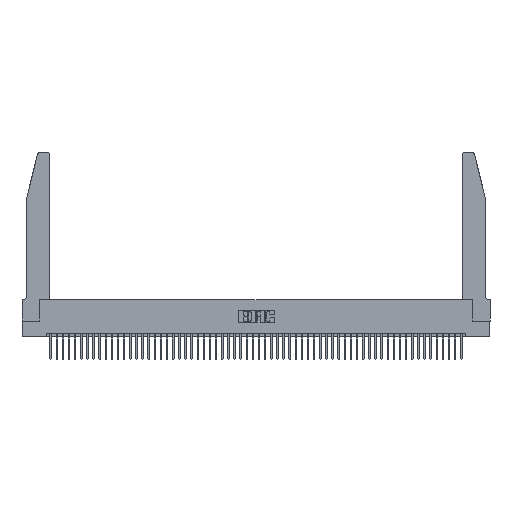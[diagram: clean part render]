
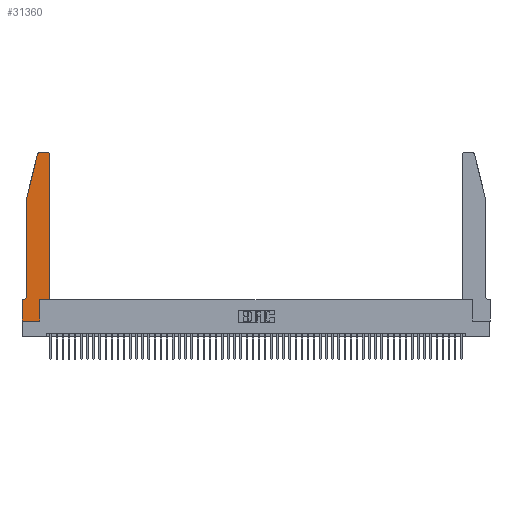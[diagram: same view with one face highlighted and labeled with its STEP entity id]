
A CAD part, top view. The second image highlights one B-rep face of the part: STEP entity #31360.
In plain terms, the highlighted planar face has unit normal (0, 0, 1).
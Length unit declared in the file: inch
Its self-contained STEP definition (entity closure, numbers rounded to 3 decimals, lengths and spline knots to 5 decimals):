
#433 = VERTEX_POINT ( 'NONE', #43734 ) ;
#1909 = ORIENTED_EDGE ( 'NONE', *, *, #45618, .T. ) ;
#3272 = FACE_OUTER_BOUND ( 'NONE', #50209, .T. ) ;
#3766 = CARTESIAN_POINT ( 'NONE',  ( 0., 0., 0.37 ) ) ;
#4046 = DIRECTION ( 'NONE',  ( 0., 0., -1. ) ) ;
#4512 = LINE ( 'NONE', #30137, #24346 ) ;
#6348 = CARTESIAN_POINT ( 'NONE',  ( 0.0755, 2., 0.37 ) ) ;
#7104 = ORIENTED_EDGE ( 'NONE', *, *, #36460, .T. ) ;
#7847 = ORIENTED_EDGE ( 'NONE', *, *, #46604, .T. ) ;
#8444 = VERTEX_POINT ( 'NONE', #13459 ) ;
#9307 = VERTEX_POINT ( 'NONE', #34593 ) ;
#9309 = VERTEX_POINT ( 'NONE', #9315 ) ;
#9315 = CARTESIAN_POINT ( 'NONE',  ( 0.4505, 2.72, 0.37 ) ) ;
#11654 = VECTOR ( 'NONE', #35386, 39.37008 ) ;
#12105 = CARTESIAN_POINT ( 'NONE',  ( 0.284, 2.72, 0.37 ) ) ;
#12354 = LINE ( 'NONE', #37042, #32099 ) ;
#13044 = CIRCLE ( 'NONE', #27682, 0.07 ) ;
#13131 = CARTESIAN_POINT ( 'NONE',  ( 0.0755, 0.42, 0.37 ) ) ;
#13279 = ORIENTED_EDGE ( 'NONE', *, *, #46031, .T. ) ;
#13411 = CARTESIAN_POINT ( 'NONE',  ( 0., 0.35, 0.37 ) ) ;
#13459 = CARTESIAN_POINT ( 'NONE',  ( 0.0055, 0.35, 0.37 ) ) ;
#13509 = VERTEX_POINT ( 'NONE', #30182 ) ;
#14500 = CARTESIAN_POINT ( 'NONE',  ( 0.0755, 2., 0.37 ) ) ;
#14809 = CARTESIAN_POINT ( 'NONE',  ( 0., 0.35, 0.37 ) ) ;
#15354 = CIRCLE ( 'NONE', #24052, 0.03 ) ;
#15947 = LINE ( 'NONE', #53700, #48142 ) ;
#16117 = VERTEX_POINT ( 'NONE', #13131 ) ;
#16398 = DIRECTION ( 'NONE',  ( 1., 0., 0. ) ) ;
#17686 = DIRECTION ( 'NONE',  ( 1., 0., 0. ) ) ;
#17772 = ORIENTED_EDGE ( 'NONE', *, *, #32910, .T. ) ;
#17981 = ORIENTED_EDGE ( 'NONE', *, *, #23582, .T. ) ;
#18593 = DIRECTION ( 'NONE',  ( 0., -1., 0. ) ) ;
#20157 = VERTEX_POINT ( 'NONE', #3766 ) ;
#20352 = LINE ( 'NONE', #6348, #41393 ) ;
#20749 = EDGE_CURVE ( 'NONE', #8444, #48089, #12354, .T. ) ;
#20758 = DIRECTION ( 'NONE',  ( 0., 1., 0. ) ) ;
#21762 = VERTEX_POINT ( 'NONE', #31262 ) ;
#21890 = CARTESIAN_POINT ( 'NONE',  ( 0.4205, 2.72, 0.37 ) ) ;
#22888 = LINE ( 'NONE', #31159, #11654 ) ;
#23380 = DIRECTION ( 'NONE',  ( -0.239, -0.971, 0. ) ) ;
#23582 = EDGE_CURVE ( 'NONE', #9309, #13509, #15354, .T. ) ;
#24052 = AXIS2_PLACEMENT_3D ( 'NONE', #21890, #51299, #26134 ) ;
#24290 = DIRECTION ( 'NONE',  ( 1., 0., 0. ) ) ;
#24346 = VECTOR ( 'NONE', #26072, 39.37008 ) ;
#24710 = CARTESIAN_POINT ( 'NONE',  ( 0.25487, 2.72718, 0.37 ) ) ;
#24776 = CARTESIAN_POINT ( 'NONE',  ( 0.4505, 0.35, 0.37 ) ) ;
#25330 = CARTESIAN_POINT ( 'NONE',  ( 0.2865, 0.35, 0.37 ) ) ;
#26072 = DIRECTION ( 'NONE',  ( 0., 1., 0. ) ) ;
#26134 = DIRECTION ( 'NONE',  ( 1., 0., 0. ) ) ;
#26458 = DIRECTION ( 'NONE',  ( -1., 0., 0. ) ) ;
#26965 = EDGE_CURVE ( 'NONE', #16117, #8444, #13044, .T. ) ;
#27682 = AXIS2_PLACEMENT_3D ( 'NONE', #29389, #4046, #33603 ) ;
#28227 = EDGE_CURVE ( 'NONE', #21762, #29455, #35266, .T. ) ;
#28673 = DIRECTION ( 'NONE',  ( 0., -1., 0. ) ) ;
#29389 = CARTESIAN_POINT ( 'NONE',  ( 0.0055, 0.42, 0.37 ) ) ;
#29439 = VECTOR ( 'NONE', #26458, 39.37008 ) ;
#29455 = VERTEX_POINT ( 'NONE', #24710 ) ;
#29719 = VECTOR ( 'NONE', #18593, 39.37008 ) ;
#30137 = CARTESIAN_POINT ( 'NONE',  ( 0.2865, 0.35, 0.37 ) ) ;
#30182 = CARTESIAN_POINT ( 'NONE',  ( 0.4205, 2.75, 0.37 ) ) ;
#31159 = CARTESIAN_POINT ( 'NONE',  ( 0.4505, 0.35, 0.37 ) ) ;
#31262 = CARTESIAN_POINT ( 'NONE',  ( 0.284, 2.75, 0.37 ) ) ;
#31360 = ADVANCED_FACE ( 'NONE', ( #3272 ), #38437, .T. ) ;
#31865 = VERTEX_POINT ( 'NONE', #25330 ) ;
#32099 = VECTOR ( 'NONE', #32987, 39.37008 ) ;
#32787 = AXIS2_PLACEMENT_3D ( 'NONE', #13411, #42874, #17686 ) ;
#32910 = EDGE_CURVE ( 'NONE', #29455, #41515, #20352, .T. ) ;
#32987 = DIRECTION ( 'NONE',  ( -1., 0., 0. ) ) ;
#33230 = ORIENTED_EDGE ( 'NONE', *, *, #48015, .T. ) ;
#33603 = DIRECTION ( 'NONE',  ( -1., 0., 0. ) ) ;
#34593 = CARTESIAN_POINT ( 'NONE',  ( 0.4505, 0.35, 0.37 ) ) ;
#35266 = CIRCLE ( 'NONE', #44283, 0.03 ) ;
#35386 = DIRECTION ( 'NONE',  ( 1., 0., 0. ) ) ;
#36460 = EDGE_CURVE ( 'NONE', #13509, #21762, #40598, .T. ) ;
#36946 = VECTOR ( 'NONE', #28673, 39.37008 ) ;
#37042 = CARTESIAN_POINT ( 'NONE',  ( 0.0755, 0.35, 0.37 ) ) ;
#38111 = ORIENTED_EDGE ( 'NONE', *, *, #41088, .T. ) ;
#38437 = PLANE ( 'NONE',  #32787 ) ;
#39474 = ORIENTED_EDGE ( 'NONE', *, *, #46416, .T. ) ;
#40236 = ORIENTED_EDGE ( 'NONE', *, *, #28227, .T. ) ;
#40598 = LINE ( 'NONE', #47390, #29439 ) ;
#41088 = EDGE_CURVE ( 'NONE', #41515, #16117, #45476, .T. ) ;
#41393 = VECTOR ( 'NONE', #23380, 39.37008 ) ;
#41515 = VERTEX_POINT ( 'NONE', #14500 ) ;
#41567 = DIRECTION ( 'NONE',  ( 0., 0., 1. ) ) ;
#42874 = DIRECTION ( 'NONE',  ( 0., 0., 1. ) ) ;
#42911 = ORIENTED_EDGE ( 'NONE', *, *, #20749, .T. ) ;
#43484 = VECTOR ( 'NONE', #20758, 39.37008 ) ;
#43734 = CARTESIAN_POINT ( 'NONE',  ( 0.2865, 0., 0.37 ) ) ;
#43784 = CARTESIAN_POINT ( 'NONE',  ( 0., 0., 0.37 ) ) ;
#44283 = AXIS2_PLACEMENT_3D ( 'NONE', #12105, #41567, #16398 ) ;
#45476 = LINE ( 'NONE', #54036, #36946 ) ;
#45618 = EDGE_CURVE ( 'NONE', #20157, #433, #15947, .T. ) ;
#46031 = EDGE_CURVE ( 'NONE', #48089, #20157, #52057, .T. ) ;
#46416 = EDGE_CURVE ( 'NONE', #9307, #9309, #54640, .T. ) ;
#46604 = EDGE_CURVE ( 'NONE', #433, #31865, #4512, .T. ) ;
#47390 = CARTESIAN_POINT ( 'NONE',  ( 0.2605, 2.75, 0.37 ) ) ;
#48015 = EDGE_CURVE ( 'NONE', #31865, #9307, #22888, .T. ) ;
#48089 = VERTEX_POINT ( 'NONE', #14809 ) ;
#48142 = VECTOR ( 'NONE', #24290, 39.37008 ) ;
#50209 = EDGE_LOOP ( 'NONE', ( #7104, #40236, #17772, #38111, #53276, #42911, #13279, #1909, #7847, #33230, #39474, #17981 ) ) ;
#51299 = DIRECTION ( 'NONE',  ( 0., 0., 1. ) ) ;
#52057 = LINE ( 'NONE', #43784, #29719 ) ;
#53276 = ORIENTED_EDGE ( 'NONE', *, *, #26965, .T. ) ;
#53700 = CARTESIAN_POINT ( 'NONE',  ( 0., 0., 0.37 ) ) ;
#54036 = CARTESIAN_POINT ( 'NONE',  ( 0.0755, 2., 0.37 ) ) ;
#54640 = LINE ( 'NONE', #24776, #43484 ) ;
